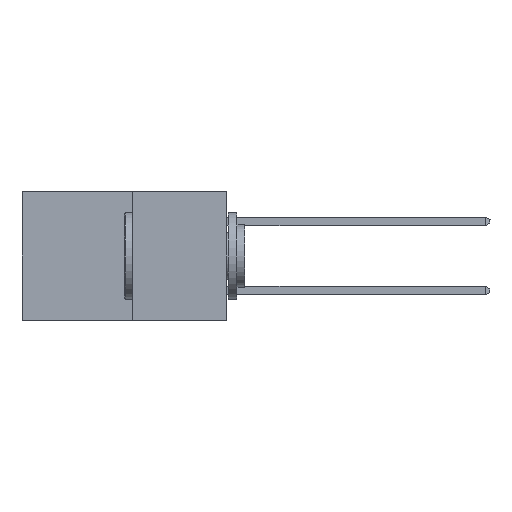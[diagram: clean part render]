
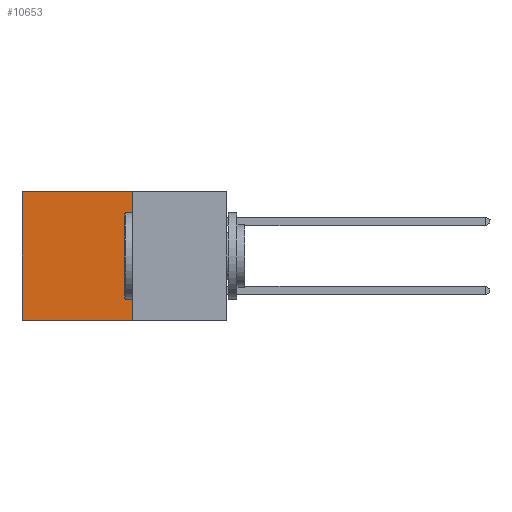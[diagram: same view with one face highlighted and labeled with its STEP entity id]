
A CAD part, left-side view. The second image highlights one B-rep face of the part: STEP entity #10653.
In plain terms, the highlighted planar face has unit normal (-1, 0, 0).
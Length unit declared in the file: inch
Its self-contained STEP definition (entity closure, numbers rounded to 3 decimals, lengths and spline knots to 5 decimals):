
#54 = CARTESIAN_POINT ( 'NONE',  ( 0.277, 0.27, -0.37 ) ) ;
#465 = ORIENTED_EDGE ( 'NONE', *, *, #2622, .F. ) ;
#1378 = DIRECTION ( 'NONE',  ( 0., 0., -1. ) ) ;
#1722 = VERTEX_POINT ( 'NONE', #5812 ) ;
#2473 = VECTOR ( 'NONE', #5001, 39.37008 ) ;
#2622 = EDGE_CURVE ( 'NONE', #5568, #1722, #9684, .T. ) ;
#3025 = EDGE_CURVE ( 'NONE', #1722, #12777, #3168, .T. ) ;
#3168 = LINE ( 'NONE', #54, #2473 ) ;
#3258 = CARTESIAN_POINT ( 'NONE',  ( 0.277, 0.27, -0.37 ) ) ;
#3863 = ORIENTED_EDGE ( 'NONE', *, *, #4919, .T. ) ;
#4919 = EDGE_CURVE ( 'NONE', #5568, #5433, #14404, .T. ) ;
#5001 = DIRECTION ( 'NONE',  ( 0., 1., 0. ) ) ;
#5433 = VERTEX_POINT ( 'NONE', #12114 ) ;
#5568 = VERTEX_POINT ( 'NONE', #6871 ) ;
#5812 = CARTESIAN_POINT ( 'NONE',  ( 0.277, 0.27, -0.37 ) ) ;
#6670 = DIRECTION ( 'NONE',  ( 1., 0., 0. ) ) ;
#6722 = VECTOR ( 'NONE', #1378, 39.37008 ) ;
#6871 = CARTESIAN_POINT ( 'NONE',  ( 0.277, 0.27, 0. ) ) ;
#7089 = VECTOR ( 'NONE', #12909, 39.37008 ) ;
#7377 = CARTESIAN_POINT ( 'NONE',  ( 0.277, 0.27, -0.37 ) ) ;
#7874 = DIRECTION ( 'NONE',  ( 0., 1., 0. ) ) ;
#8287 = CARTESIAN_POINT ( 'NONE',  ( 0.277, 0.27, 0. ) ) ;
#9141 = ORIENTED_EDGE ( 'NONE', *, *, #3025, .F. ) ;
#9684 = LINE ( 'NONE', #7377, #6722 ) ;
#10395 = LINE ( 'NONE', #11784, #7089 ) ;
#10487 = FACE_OUTER_BOUND ( 'NONE', #13725, .T. ) ;
#10653 = ADVANCED_FACE ( 'NONE', ( #10487 ), #12221, .F. ) ;
#11473 = VECTOR ( 'NONE', #7874, 39.37008 ) ;
#11753 = ORIENTED_EDGE ( 'NONE', *, *, #13766, .T. ) ;
#11784 = CARTESIAN_POINT ( 'NONE',  ( 0.277, 0.59, -0.37 ) ) ;
#12114 = CARTESIAN_POINT ( 'NONE',  ( 0.277, 0.59, 0. ) ) ;
#12221 = PLANE ( 'NONE',  #12260 ) ;
#12260 = AXIS2_PLACEMENT_3D ( 'NONE', #3258, #6670, #14422 ) ;
#12777 = VERTEX_POINT ( 'NONE', #13508 ) ;
#12909 = DIRECTION ( 'NONE',  ( 0., 0., -1. ) ) ;
#13508 = CARTESIAN_POINT ( 'NONE',  ( 0.277, 0.59, -0.37 ) ) ;
#13725 = EDGE_LOOP ( 'NONE', ( #11753, #9141, #465, #3863 ) ) ;
#13766 = EDGE_CURVE ( 'NONE', #5433, #12777, #10395, .T. ) ;
#14404 = LINE ( 'NONE', #8287, #11473 ) ;
#14422 = DIRECTION ( 'NONE',  ( 0., 0., -1. ) ) ;
